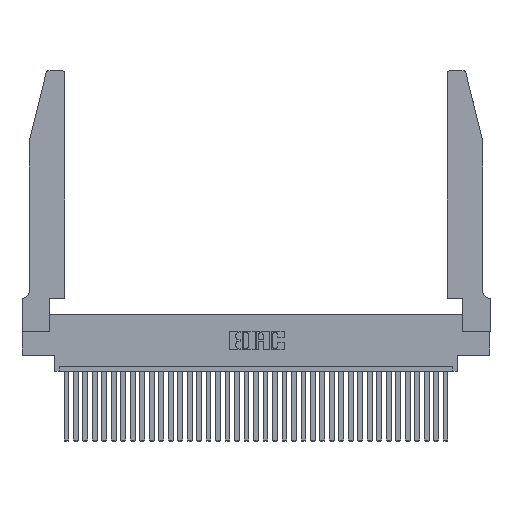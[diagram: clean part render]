
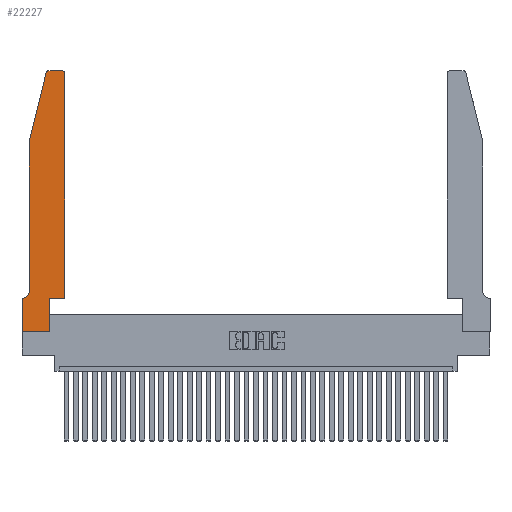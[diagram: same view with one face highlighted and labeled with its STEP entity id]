
A CAD part, top view. The second image highlights one B-rep face of the part: STEP entity #22227.
In plain terms, the highlighted planar face has unit normal (0, 0, 1).
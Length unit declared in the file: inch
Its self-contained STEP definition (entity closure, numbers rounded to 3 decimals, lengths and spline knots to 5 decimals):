
#557 = DIRECTION ( 'NONE',  ( 1., 0., 0. ) ) ;
#1298 = VERTEX_POINT ( 'NONE', #12204 ) ;
#1401 = AXIS2_PLACEMENT_3D ( 'NONE', #27372, #13825, #18764 ) ;
#1614 = DIRECTION ( 'NONE',  ( 0., -1., 0. ) ) ;
#1987 = DIRECTION ( 'NONE',  ( 1., 0., 0. ) ) ;
#2597 = DIRECTION ( 'NONE',  ( 1., 0., 0. ) ) ;
#3091 = CARTESIAN_POINT ( 'NONE',  ( 0., 0., 0.37 ) ) ;
#3426 = LINE ( 'NONE', #17648, #33225 ) ;
#3492 = CARTESIAN_POINT ( 'NONE',  ( 0.0755, 0.35, 0.37 ) ) ;
#3535 = CARTESIAN_POINT ( 'NONE',  ( 0.25487, 2.72718, 0.37 ) ) ;
#4172 = CARTESIAN_POINT ( 'NONE',  ( 0.2865, 0., 0.37 ) ) ;
#4310 = CARTESIAN_POINT ( 'NONE',  ( 0.0755, 0.42, 0.37 ) ) ;
#4426 = LINE ( 'NONE', #3492, #10920 ) ;
#4436 = DIRECTION ( 'NONE',  ( -1., 0., 0. ) ) ;
#4507 = ORIENTED_EDGE ( 'NONE', *, *, #30457, .T. ) ;
#5467 = CARTESIAN_POINT ( 'NONE',  ( 0.0755, 2., 0.37 ) ) ;
#5807 = VERTEX_POINT ( 'NONE', #24534 ) ;
#5949 = LINE ( 'NONE', #33654, #12003 ) ;
#5966 = ORIENTED_EDGE ( 'NONE', *, *, #15128, .T. ) ;
#6189 = AXIS2_PLACEMENT_3D ( 'NONE', #32167, #35027, #29285 ) ;
#6206 = ORIENTED_EDGE ( 'NONE', *, *, #35463, .T. ) ;
#7297 = CARTESIAN_POINT ( 'NONE',  ( 0.2865, 0.35, 0.37 ) ) ;
#7336 = DIRECTION ( 'NONE',  ( 0., 0., 1. ) ) ;
#7509 = VERTEX_POINT ( 'NONE', #4310 ) ;
#8751 = ORIENTED_EDGE ( 'NONE', *, *, #22013, .T. ) ;
#9498 = VECTOR ( 'NONE', #20064, 39.37008 ) ;
#9962 = CARTESIAN_POINT ( 'NONE',  ( 0.4205, 2.72, 0.37 ) ) ;
#10250 = DIRECTION ( 'NONE',  ( 1., 0., 0. ) ) ;
#10366 = EDGE_CURVE ( 'NONE', #28644, #7509, #16400, .T. ) ;
#10920 = VECTOR ( 'NONE', #31122, 39.37008 ) ;
#11322 = EDGE_CURVE ( 'NONE', #20210, #31109, #12871, .T. ) ;
#12003 = VECTOR ( 'NONE', #20276, 39.37008 ) ;
#12041 = AXIS2_PLACEMENT_3D ( 'NONE', #26816, #7336, #10250 ) ;
#12204 = CARTESIAN_POINT ( 'NONE',  ( 0.4505, 0.35, 0.37 ) ) ;
#12766 = DIRECTION ( 'NONE',  ( 0., 0., 1. ) ) ;
#12818 = ORIENTED_EDGE ( 'NONE', *, *, #23131, .T. ) ;
#12871 = CIRCLE ( 'NONE', #27357, 0.03 ) ;
#13686 = LINE ( 'NONE', #35159, #14566 ) ;
#13825 = DIRECTION ( 'NONE',  ( 0., 0., -1. ) ) ;
#13996 = EDGE_CURVE ( 'NONE', #33591, #28644, #3426, .T. ) ;
#14566 = VECTOR ( 'NONE', #4436, 39.37008 ) ;
#14644 = VECTOR ( 'NONE', #1614, 39.37008 ) ;
#14828 = CARTESIAN_POINT ( 'NONE',  ( 0.0755, 2., 0.37 ) ) ;
#15128 = EDGE_CURVE ( 'NONE', #1298, #20210, #5949, .T. ) ;
#15304 = CARTESIAN_POINT ( 'NONE',  ( 0., 0., 0.37 ) ) ;
#15779 = ORIENTED_EDGE ( 'NONE', *, *, #35633, .T. ) ;
#16400 = LINE ( 'NONE', #14828, #27662 ) ;
#16775 = CARTESIAN_POINT ( 'NONE',  ( 0.284, 2.75, 0.37 ) ) ;
#16981 = VECTOR ( 'NONE', #557, 39.37008 ) ;
#17648 = CARTESIAN_POINT ( 'NONE',  ( 0.0755, 2., 0.37 ) ) ;
#18764 = DIRECTION ( 'NONE',  ( -1., 0., 0. ) ) ;
#19773 = CARTESIAN_POINT ( 'NONE',  ( 0.4505, 0.35, 0.37 ) ) ;
#20064 = DIRECTION ( 'NONE',  ( 0., 1., 0. ) ) ;
#20210 = VERTEX_POINT ( 'NONE', #21912 ) ;
#20276 = DIRECTION ( 'NONE',  ( 0., 1., 0. ) ) ;
#20981 = EDGE_CURVE ( 'NONE', #31109, #23204, #13686, .T. ) ;
#21912 = CARTESIAN_POINT ( 'NONE',  ( 0.4505, 2.72, 0.37 ) ) ;
#22008 = VECTOR ( 'NONE', #2597, 39.37008 ) ;
#22013 = EDGE_CURVE ( 'NONE', #7509, #35478, #34714, .T. ) ;
#22227 = ADVANCED_FACE ( 'NONE', ( #23490 ), #32075, .T. ) ;
#22616 = VERTEX_POINT ( 'NONE', #33953 ) ;
#23131 = EDGE_CURVE ( 'NONE', #22616, #1298, #23423, .T. ) ;
#23196 = VERTEX_POINT ( 'NONE', #4172 ) ;
#23204 = VERTEX_POINT ( 'NONE', #16775 ) ;
#23423 = LINE ( 'NONE', #19773, #16981 ) ;
#23476 = DIRECTION ( 'NONE',  ( 0., -1., 0. ) ) ;
#23490 = FACE_OUTER_BOUND ( 'NONE', #32935, .T. ) ;
#23667 = DIRECTION ( 'NONE',  ( -0.239, -0.971, 0. ) ) ;
#24293 = VERTEX_POINT ( 'NONE', #15304 ) ;
#24534 = CARTESIAN_POINT ( 'NONE',  ( 0., 0.35, 0.37 ) ) ;
#25020 = LINE ( 'NONE', #30354, #22008 ) ;
#26208 = EDGE_CURVE ( 'NONE', #5807, #24293, #27180, .T. ) ;
#26816 = CARTESIAN_POINT ( 'NONE',  ( 0., 0.35, 0.37 ) ) ;
#26958 = ORIENTED_EDGE ( 'NONE', *, *, #11322, .T. ) ;
#27180 = LINE ( 'NONE', #3091, #14644 ) ;
#27261 = ORIENTED_EDGE ( 'NONE', *, *, #20981, .T. ) ;
#27357 = AXIS2_PLACEMENT_3D ( 'NONE', #9962, #12766, #1987 ) ;
#27372 = CARTESIAN_POINT ( 'NONE',  ( 0.0055, 0.42, 0.37 ) ) ;
#27662 = VECTOR ( 'NONE', #23476, 39.37008 ) ;
#28005 = ORIENTED_EDGE ( 'NONE', *, *, #33871, .T. ) ;
#28644 = VERTEX_POINT ( 'NONE', #5467 ) ;
#29040 = ORIENTED_EDGE ( 'NONE', *, *, #13996, .T. ) ;
#29285 = DIRECTION ( 'NONE',  ( 1., 0., 0. ) ) ;
#29525 = CARTESIAN_POINT ( 'NONE',  ( 0.0055, 0.35, 0.37 ) ) ;
#29683 = ORIENTED_EDGE ( 'NONE', *, *, #10366, .T. ) ;
#29741 = CIRCLE ( 'NONE', #6189, 0.03 ) ;
#30354 = CARTESIAN_POINT ( 'NONE',  ( 0., 0., 0.37 ) ) ;
#30457 = EDGE_CURVE ( 'NONE', #23196, #22616, #32797, .T. ) ;
#30742 = ORIENTED_EDGE ( 'NONE', *, *, #26208, .T. ) ;
#31109 = VERTEX_POINT ( 'NONE', #34289 ) ;
#31122 = DIRECTION ( 'NONE',  ( -1., 0., 0. ) ) ;
#32075 = PLANE ( 'NONE',  #12041 ) ;
#32167 = CARTESIAN_POINT ( 'NONE',  ( 0.284, 2.72, 0.37 ) ) ;
#32797 = LINE ( 'NONE', #7297, #9498 ) ;
#32935 = EDGE_LOOP ( 'NONE', ( #27261, #6206, #29040, #29683, #8751, #28005, #30742, #15779, #4507, #12818, #5966, #26958 ) ) ;
#33225 = VECTOR ( 'NONE', #23667, 39.37008 ) ;
#33591 = VERTEX_POINT ( 'NONE', #3535 ) ;
#33654 = CARTESIAN_POINT ( 'NONE',  ( 0.4505, 0.35, 0.37 ) ) ;
#33871 = EDGE_CURVE ( 'NONE', #35478, #5807, #4426, .T. ) ;
#33953 = CARTESIAN_POINT ( 'NONE',  ( 0.2865, 0.35, 0.37 ) ) ;
#34289 = CARTESIAN_POINT ( 'NONE',  ( 0.4205, 2.75, 0.37 ) ) ;
#34714 = CIRCLE ( 'NONE', #1401, 0.07 ) ;
#35027 = DIRECTION ( 'NONE',  ( 0., 0., 1. ) ) ;
#35159 = CARTESIAN_POINT ( 'NONE',  ( 0.2605, 2.75, 0.37 ) ) ;
#35463 = EDGE_CURVE ( 'NONE', #23204, #33591, #29741, .T. ) ;
#35478 = VERTEX_POINT ( 'NONE', #29525 ) ;
#35633 = EDGE_CURVE ( 'NONE', #24293, #23196, #25020, .T. ) ;
